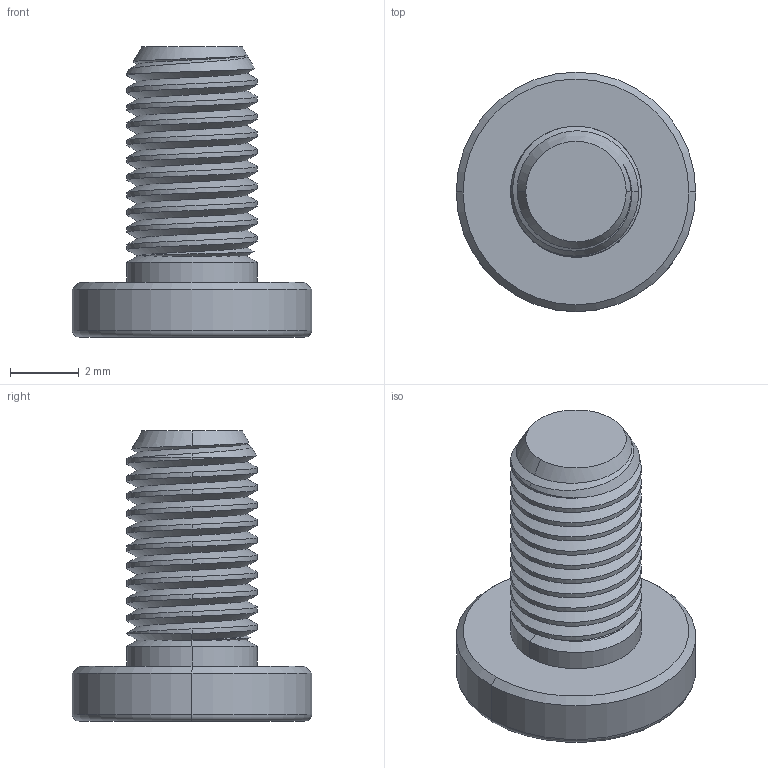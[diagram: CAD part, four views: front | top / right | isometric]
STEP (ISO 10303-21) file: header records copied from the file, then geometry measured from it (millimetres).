
FILE_DESCRIPTION (( 'STEP AP214' ), '1' );
FILE_NAME ('Schraube_Griffstück.STEP', '2013-07-30T15:11:09', ( 'Asher' ), ( '' ), 'SwSTEP 2.0', 'SolidWorks 2013', '' );
FILE_SCHEMA (( 'AUTOMOTIVE_DESIGN' ));
Length unit declared in the file: millimetre
Products named in the file (1): Schraube_Griffstück
Bounding box: 6.99 x 6.99 x 8.46 mm (x, y, z)
Volume: 112.7 mm3; surface area: 243.4 mm2
Topology: 1 solids, 1 shells, 56 faces, 138 edges, 86 vertices
Faces by surface type: cylinder 26, plane 16, cone 10, torus 2, bspline 2
Entity records: 2665 total; most frequent: CARTESIAN_POINT 1448, ORIENTED_EDGE 276, DIRECTION 217, EDGE_CURVE 138, VERTEX_POINT 86, AXIS2_PLACEMENT_3D 76, VECTOR 65, LINE 65
